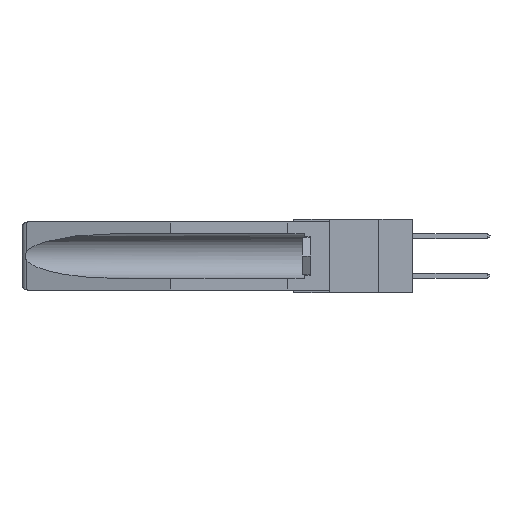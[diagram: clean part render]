
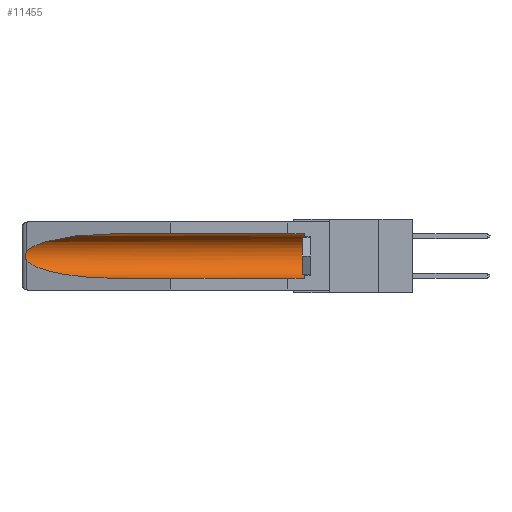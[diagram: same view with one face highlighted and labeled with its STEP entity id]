
A CAD part, left-side view. The second image highlights one B-rep face of the part: STEP entity #11455.
In plain terms, the highlighted cylindrical face has radius 2.857 mm (diameter 5.715 mm), a partial arc.
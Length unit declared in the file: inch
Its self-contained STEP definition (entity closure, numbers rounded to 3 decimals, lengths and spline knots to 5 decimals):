
#29 = CARTESIAN_POINT ( 'NONE',  ( 0.155, 1.07973, -0.284 ) ) ;
#108 = CARTESIAN_POINT ( 'NONE',  ( 0.26537, 1.52718, -0.14972 ) ) ;
#392 = EDGE_CURVE ( 'NONE', #3581, #12627, #22835, .T. ) ;
#434 = CARTESIAN_POINT ( 'NONE',  ( 0.26537, 1.52718, -0.19328 ) ) ;
#1383 = EDGE_CURVE ( 'NONE', #20763, #16925, #4561, .T. ) ;
#2592 = EDGE_CURVE ( 'NONE', #3581, #7711, #21823, .T. ) ;
#2714 = CARTESIAN_POINT ( 'NONE',  ( 0.155, 1.07973, -0.284 ) ) ;
#2719 = ORIENTED_EDGE ( 'NONE', *, *, #2592, .F. ) ;
#2811 = DIRECTION ( 'NONE',  ( 0., 1., 0. ) ) ;
#3405 = CARTESIAN_POINT ( 'NONE',  ( 0.2675, 1.53308, -0.17534 ) ) ;
#3431 = CARTESIAN_POINT ( 'NONE',  ( 0.155, 0.126, -0.059 ) ) ;
#3486 = CARTESIAN_POINT ( 'NONE',  ( 0.2673, 1.53269, -0.17917 ) ) ;
#3581 = VERTEX_POINT ( 'NONE', #21173 ) ;
#3715 = EDGE_CURVE ( 'NONE', #12627, #22611, #15395, .T. ) ;
#4324 = VECTOR ( 'NONE', #2811, 39.37008 ) ;
#4561 = B_SPLINE_CURVE_WITH_KNOTS ( 'NONE', 3,
 ( #108, #12559, #8810, #10521, #14322, #3405, #3486, #15947, #14029, #17795 ),
 .UNSPECIFIED., .F., .F.,
 ( 4, 2, 2, 2, 4 ),
 ( 0., 0.00029, 0.00058, 0.00087, 0.00117 ),
 .UNSPECIFIED. ) ;
#4666 = CARTESIAN_POINT ( 'NONE',  ( 0.21114, 1.30732, -0.284 ) ) ;
#4754 = EDGE_CURVE ( 'NONE', #22611, #20763, #5239, .T. ) ;
#5239 =( BOUNDED_CURVE ( )  B_SPLINE_CURVE ( 3, ( #7798, #21674, #14629, #19956 ),
 .UNSPECIFIED., .F., .F. ) 
 B_SPLINE_CURVE_WITH_KNOTS ( ( 4, 4 ),
 ( 4.71239, 6.08839 ),
 .UNSPECIFIED. ) 
 CURVE ( )  GEOMETRIC_REPRESENTATION_ITEM ( )  RATIONAL_B_SPLINE_CURVE ( ( 1., 0.848, 0.848, 1. ) ) 
 REPRESENTATION_ITEM ( '' )  );
#5343 = DIRECTION ( 'NONE',  ( 0., 0., 1. ) ) ;
#6555 = CARTESIAN_POINT ( 'NONE',  ( 0.155, -0.30754, -0.284 ) ) ;
#7248 = DIRECTION ( 'NONE',  ( 0., 0., 1. ) ) ;
#7711 = VERTEX_POINT ( 'NONE', #29 ) ;
#7798 = CARTESIAN_POINT ( 'NONE',  ( 0.155, 1.07973, -0.059 ) ) ;
#8810 = CARTESIAN_POINT ( 'NONE',  ( 0.26654, 1.53092, -0.15636 ) ) ;
#8880 = ORIENTED_EDGE ( 'NONE', *, *, #17084, .T. ) ;
#8883 = EDGE_LOOP ( 'NONE', ( #15595, #11968, #8880, #2719, #19593, #18576 ) ) ;
#9763 = CARTESIAN_POINT ( 'NONE',  ( 0.155, -0.30754, -0.059 ) ) ;
#10521 = CARTESIAN_POINT ( 'NONE',  ( 0.2673, 1.5327, -0.16383 ) ) ;
#11455 = ADVANCED_FACE ( 'NONE', ( #17600 ), #21774, .F. ) ;
#11968 = ORIENTED_EDGE ( 'NONE', *, *, #1383, .T. ) ;
#12390 = DIRECTION ( 'NONE',  ( 0., -1., 0. ) ) ;
#12559 = CARTESIAN_POINT ( 'NONE',  ( 0.26597, 1.52961, -0.15275 ) ) ;
#12627 = VERTEX_POINT ( 'NONE', #3431 ) ;
#14029 = CARTESIAN_POINT ( 'NONE',  ( 0.26597, 1.5296, -0.19026 ) ) ;
#14322 = CARTESIAN_POINT ( 'NONE',  ( 0.2675, 1.53308, -0.16763 ) ) ;
#14448 = CARTESIAN_POINT ( 'NONE',  ( 0.26537, 1.52718, -0.14972 ) ) ;
#14620 = CARTESIAN_POINT ( 'NONE',  ( 0.155, 1.07973, -0.059 ) ) ;
#14627 = VECTOR ( 'NONE', #22654, 39.37008 ) ;
#14629 = CARTESIAN_POINT ( 'NONE',  ( 0.25451, 1.48313, -0.09465 ) ) ;
#14940 = CARTESIAN_POINT ( 'NONE',  ( 0.26537, 1.52718, -0.19328 ) ) ;
#15220 = AXIS2_PLACEMENT_3D ( 'NONE', #22842, #17638, #5343 ) ;
#15395 = LINE ( 'NONE', #9763, #4324 ) ;
#15595 = ORIENTED_EDGE ( 'NONE', *, *, #4754, .T. ) ;
#15875 =( BOUNDED_CURVE ( )  B_SPLINE_CURVE ( 3, ( #14940, #20283, #4666, #2714 ),
 .UNSPECIFIED., .F., .F. ) 
 B_SPLINE_CURVE_WITH_KNOTS ( ( 4, 4 ),
 ( 0.1948, 1.5708 ),
 .UNSPECIFIED. ) 
 CURVE ( )  GEOMETRIC_REPRESENTATION_ITEM ( )  RATIONAL_B_SPLINE_CURVE ( ( 1., 0.848, 0.848, 1. ) ) 
 REPRESENTATION_ITEM ( '' )  );
#15947 = CARTESIAN_POINT ( 'NONE',  ( 0.26655, 1.53094, -0.18657 ) ) ;
#16925 = VERTEX_POINT ( 'NONE', #434 ) ;
#17084 = EDGE_CURVE ( 'NONE', #16925, #7711, #15875, .T. ) ;
#17600 = FACE_OUTER_BOUND ( 'NONE', #8883, .T. ) ;
#17620 = CARTESIAN_POINT ( 'NONE',  ( 0.155, 0.126, -0.1715 ) ) ;
#17638 = DIRECTION ( 'NONE',  ( 0., 1., 0. ) ) ;
#17795 = CARTESIAN_POINT ( 'NONE',  ( 0.26537, 1.52718, -0.19328 ) ) ;
#18576 = ORIENTED_EDGE ( 'NONE', *, *, #3715, .T. ) ;
#19593 = ORIENTED_EDGE ( 'NONE', *, *, #392, .T. ) ;
#19956 = CARTESIAN_POINT ( 'NONE',  ( 0.26537, 1.52718, -0.14972 ) ) ;
#20098 = AXIS2_PLACEMENT_3D ( 'NONE', #17620, #12390, #7248 ) ;
#20283 = CARTESIAN_POINT ( 'NONE',  ( 0.25451, 1.48313, -0.24835 ) ) ;
#20763 = VERTEX_POINT ( 'NONE', #14448 ) ;
#21173 = CARTESIAN_POINT ( 'NONE',  ( 0.155, 0.126, -0.284 ) ) ;
#21674 = CARTESIAN_POINT ( 'NONE',  ( 0.21114, 1.30732, -0.059 ) ) ;
#21774 = CYLINDRICAL_SURFACE ( 'NONE', #15220, 0.1125 ) ;
#21823 = LINE ( 'NONE', #6555, #14627 ) ;
#22611 = VERTEX_POINT ( 'NONE', #14620 ) ;
#22654 = DIRECTION ( 'NONE',  ( 0., 1., 0. ) ) ;
#22835 = CIRCLE ( 'NONE', #20098, 0.1125 ) ;
#22842 = CARTESIAN_POINT ( 'NONE',  ( 0.155, -0.30754, -0.1715 ) ) ;
